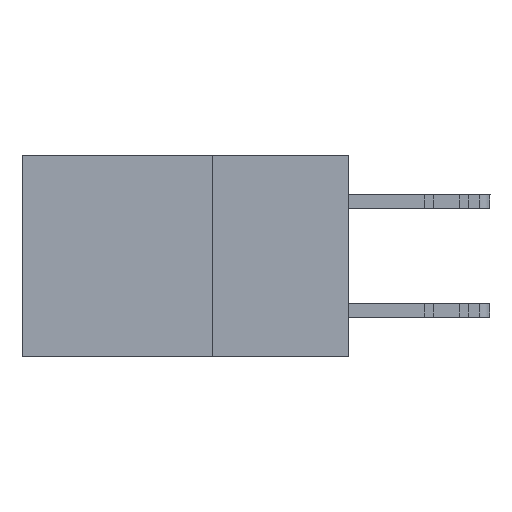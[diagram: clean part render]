
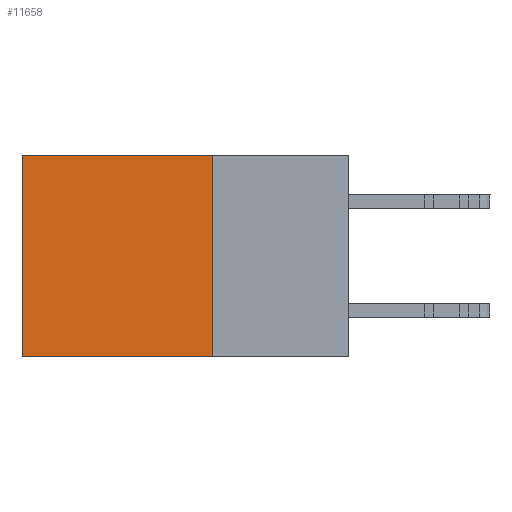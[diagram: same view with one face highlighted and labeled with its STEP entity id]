
A CAD part, left-side view. The second image highlights one B-rep face of the part: STEP entity #11658.
In plain terms, the highlighted planar face has unit normal (-1, 0, 0).
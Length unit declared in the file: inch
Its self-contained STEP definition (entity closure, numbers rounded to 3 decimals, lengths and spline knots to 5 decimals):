
#862 = CARTESIAN_POINT ( 'NONE',  ( 0.298, 0.25, -0.37 ) ) ;
#2245 = VERTEX_POINT ( 'NONE', #20547 ) ;
#3553 = AXIS2_PLACEMENT_3D ( 'NONE', #27289, #20109, #9102 ) ;
#3945 = EDGE_CURVE ( 'NONE', #2245, #24651, #5067, .T. ) ;
#5067 = LINE ( 'NONE', #25026, #20096 ) ;
#6786 = PLANE ( 'NONE',  #3553 ) ;
#7077 = VERTEX_POINT ( 'NONE', #862 ) ;
#7227 = CARTESIAN_POINT ( 'NONE',  ( 0.298, 0.6, 0. ) ) ;
#8364 = EDGE_CURVE ( 'NONE', #24651, #17189, #18228, .T. ) ;
#8631 = DIRECTION ( 'NONE',  ( 0., 0., -1. ) ) ;
#9102 = DIRECTION ( 'NONE',  ( 0., 0., -1. ) ) ;
#9691 = DIRECTION ( 'NONE',  ( 0., 1., 0. ) ) ;
#10473 = EDGE_CURVE ( 'NONE', #7077, #17189, #11404, .T. ) ;
#10774 = CARTESIAN_POINT ( 'NONE',  ( 0.298, 0.25, 0. ) ) ;
#11404 = LINE ( 'NONE', #20267, #12787 ) ;
#11658 = ADVANCED_FACE ( 'NONE', ( #22942 ), #6786, .F. ) ;
#11793 = ORIENTED_EDGE ( 'NONE', *, *, #26408, .F. ) ;
#12416 = DIRECTION ( 'NONE',  ( 0., 1., 0. ) ) ;
#12787 = VECTOR ( 'NONE', #12416, 39.37008 ) ;
#13378 = VECTOR ( 'NONE', #8631, 39.37008 ) ;
#15270 = LINE ( 'NONE', #10774, #13378 ) ;
#15779 = EDGE_LOOP ( 'NONE', ( #24429, #20586, #11793, #26926 ) ) ;
#17189 = VERTEX_POINT ( 'NONE', #22282 ) ;
#18228 = LINE ( 'NONE', #7227, #23390 ) ;
#19201 = CARTESIAN_POINT ( 'NONE',  ( 0.298, 0.6, 0. ) ) ;
#20096 = VECTOR ( 'NONE', #9691, 39.37008 ) ;
#20109 = DIRECTION ( 'NONE',  ( 1., 0., 0. ) ) ;
#20267 = CARTESIAN_POINT ( 'NONE',  ( 0.298, 0.25, -0.37 ) ) ;
#20547 = CARTESIAN_POINT ( 'NONE',  ( 0.298, 0.25, 0. ) ) ;
#20586 = ORIENTED_EDGE ( 'NONE', *, *, #10473, .F. ) ;
#22282 = CARTESIAN_POINT ( 'NONE',  ( 0.298, 0.6, -0.37 ) ) ;
#22942 = FACE_OUTER_BOUND ( 'NONE', #15779, .T. ) ;
#23390 = VECTOR ( 'NONE', #24880, 39.37008 ) ;
#24429 = ORIENTED_EDGE ( 'NONE', *, *, #8364, .T. ) ;
#24651 = VERTEX_POINT ( 'NONE', #19201 ) ;
#24880 = DIRECTION ( 'NONE',  ( 0., 0., -1. ) ) ;
#25026 = CARTESIAN_POINT ( 'NONE',  ( 0.298, 0.25, 0. ) ) ;
#26408 = EDGE_CURVE ( 'NONE', #2245, #7077, #15270, .T. ) ;
#26926 = ORIENTED_EDGE ( 'NONE', *, *, #3945, .T. ) ;
#27289 = CARTESIAN_POINT ( 'NONE',  ( 0.298, 0.25, 0. ) ) ;
